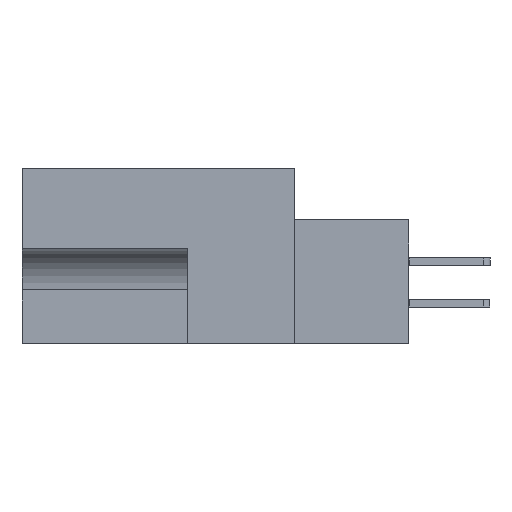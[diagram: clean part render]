
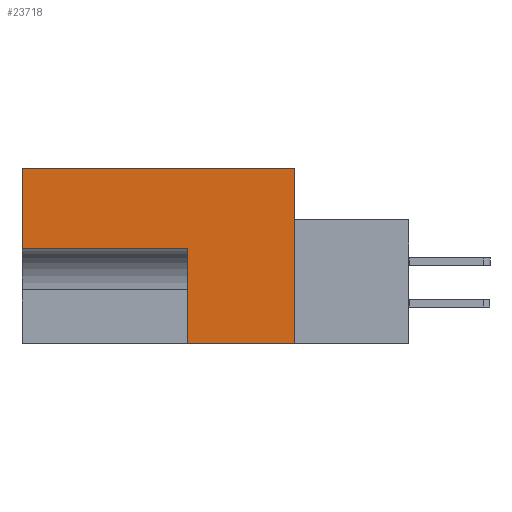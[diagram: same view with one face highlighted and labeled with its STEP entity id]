
A CAD part, left-side view. The second image highlights one B-rep face of the part: STEP entity #23718.
In plain terms, the highlighted planar face has unit normal (-1, 0, 0).
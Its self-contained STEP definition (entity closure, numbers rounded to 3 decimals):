
#381 = DIRECTION ( 'NONE',  ( 0., 0., -1. ) ) ;
#784 = VECTOR ( 'NONE', #7618, 1000. ) ;
#1074 = LINE ( 'NONE', #4063, #784 ) ;
#1123 = VERTEX_POINT ( 'NONE', #7332 ) ;
#3365 = ORIENTED_EDGE ( 'NONE', *, *, #8952, .F. ) ;
#4063 = CARTESIAN_POINT ( 'NONE',  ( 0., -8.814, -13.487 ) ) ;
#4190 = ORIENTED_EDGE ( 'NONE', *, *, #22375, .F. ) ;
#4642 = EDGE_CURVE ( 'NONE', #4856, #5665, #16785, .T. ) ;
#4767 = CARTESIAN_POINT ( 'NONE',  ( 0., 0., 0. ) ) ;
#4856 = VERTEX_POINT ( 'NONE', #22527 ) ;
#5507 = ORIENTED_EDGE ( 'NONE', *, *, #4642, .F. ) ;
#5665 = VERTEX_POINT ( 'NONE', #4767 ) ;
#5919 = DIRECTION ( 'NONE',  ( 0., 0., 1. ) ) ;
#5997 = DIRECTION ( 'NONE',  ( 1., 0., 0. ) ) ;
#6341 = LINE ( 'NONE', #19348, #9871 ) ;
#6471 = LINE ( 'NONE', #7410, #20650 ) ;
#6603 = CARTESIAN_POINT ( 'NONE',  ( 0., 0., 0. ) ) ;
#7254 = VERTEX_POINT ( 'NONE', #22182 ) ;
#7332 = CARTESIAN_POINT ( 'NONE',  ( 0., 20.955, -6.172 ) ) ;
#7410 = CARTESIAN_POINT ( 'NONE',  ( 0., 8.255, -6.172 ) ) ;
#7618 = DIRECTION ( 'NONE',  ( 0., 1., 0. ) ) ;
#8007 = DIRECTION ( 'NONE',  ( 0., 0., 1. ) ) ;
#8952 = EDGE_CURVE ( 'NONE', #5665, #10025, #9090, .T. ) ;
#9090 = LINE ( 'NONE', #17722, #23625 ) ;
#9470 = VERTEX_POINT ( 'NONE', #21593 ) ;
#9871 = VECTOR ( 'NONE', #8007, 1000. ) ;
#9946 = EDGE_CURVE ( 'NONE', #1123, #4856, #18271, .T. ) ;
#10025 = VERTEX_POINT ( 'NONE', #11380 ) ;
#10452 = AXIS2_PLACEMENT_3D ( 'NONE', #6603, #5997, #381 ) ;
#11165 = VECTOR ( 'NONE', #17815, 1000. ) ;
#11325 = ORIENTED_EDGE ( 'NONE', *, *, #20615, .F. ) ;
#11380 = CARTESIAN_POINT ( 'NONE',  ( 0., 0., -13.487 ) ) ;
#11459 = CARTESIAN_POINT ( 'NONE',  ( 0., 20.955, -13.487 ) ) ;
#11944 = FACE_OUTER_BOUND ( 'NONE', #15318, .T. ) ;
#12500 = EDGE_CURVE ( 'NONE', #7254, #9470, #6341, .T. ) ;
#13230 = VECTOR ( 'NONE', #5919, 1000. ) ;
#15318 = EDGE_LOOP ( 'NONE', ( #4190, #3365, #5507, #15540, #11325, #15950 ) ) ;
#15540 = ORIENTED_EDGE ( 'NONE', *, *, #9946, .F. ) ;
#15950 = ORIENTED_EDGE ( 'NONE', *, *, #12500, .F. ) ;
#16674 = DIRECTION ( 'NONE',  ( 0., 1., 0. ) ) ;
#16785 = LINE ( 'NONE', #19878, #11165 ) ;
#17722 = CARTESIAN_POINT ( 'NONE',  ( 0., 0., 0. ) ) ;
#17815 = DIRECTION ( 'NONE',  ( 0., -1., 0. ) ) ;
#18271 = LINE ( 'NONE', #11459, #13230 ) ;
#19242 = PLANE ( 'NONE',  #10452 ) ;
#19348 = CARTESIAN_POINT ( 'NONE',  ( 0., 8.255, -13.487 ) ) ;
#19616 = DIRECTION ( 'NONE',  ( 0., 0., -1. ) ) ;
#19878 = CARTESIAN_POINT ( 'NONE',  ( 0., 11.506, 0. ) ) ;
#20615 = EDGE_CURVE ( 'NONE', #9470, #1123, #6471, .T. ) ;
#20650 = VECTOR ( 'NONE', #16674, 1000. ) ;
#21593 = CARTESIAN_POINT ( 'NONE',  ( 0., 8.255, -6.172 ) ) ;
#22182 = CARTESIAN_POINT ( 'NONE',  ( 0., 8.255, -13.487 ) ) ;
#22375 = EDGE_CURVE ( 'NONE', #10025, #7254, #1074, .T. ) ;
#22527 = CARTESIAN_POINT ( 'NONE',  ( 0., 20.955, 0. ) ) ;
#23625 = VECTOR ( 'NONE', #19616, 1000. ) ;
#23718 = ADVANCED_FACE ( 'NONE', ( #11944 ), #19242, .F. ) ;
